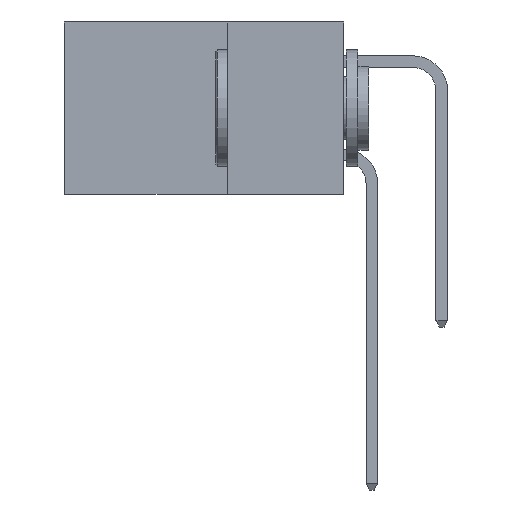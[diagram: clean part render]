
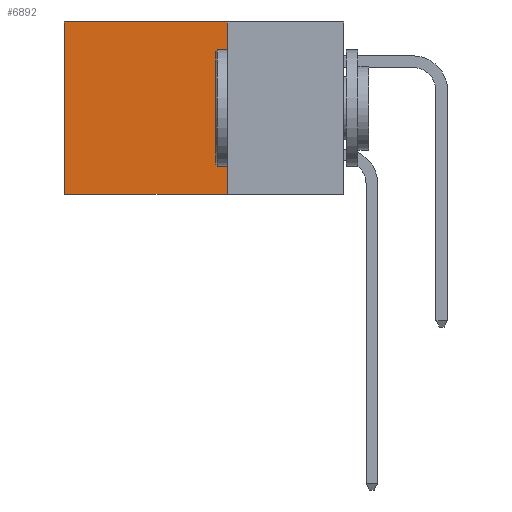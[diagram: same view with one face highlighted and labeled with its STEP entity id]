
A CAD part, left-side view. The second image highlights one B-rep face of the part: STEP entity #6892.
In plain terms, the highlighted planar face has unit normal (-1, 0, 0).
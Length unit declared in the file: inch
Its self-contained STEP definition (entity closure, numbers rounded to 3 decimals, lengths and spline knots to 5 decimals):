
#18 = PLANE ( 'NONE',  #6084 ) ;
#218 = CARTESIAN_POINT ( 'NONE',  ( 0.2615, 0.6, -0.37 ) ) ;
#992 = DIRECTION ( 'NONE',  ( 0., 0., -1. ) ) ;
#1005 = LINE ( 'NONE', #12203, #17346 ) ;
#1094 = EDGE_CURVE ( 'NONE', #1504, #15524, #16859, .T. ) ;
#1504 = VERTEX_POINT ( 'NONE', #9074 ) ;
#2095 = DIRECTION ( 'NONE',  ( 0., 0., -1. ) ) ;
#2265 = ORIENTED_EDGE ( 'NONE', *, *, #1094, .F. ) ;
#3482 = ORIENTED_EDGE ( 'NONE', *, *, #8745, .T. ) ;
#4600 = CARTESIAN_POINT ( 'NONE',  ( 0.2615, 0.25, -0.37 ) ) ;
#5393 = FACE_OUTER_BOUND ( 'NONE', #13277, .T. ) ;
#5619 = CARTESIAN_POINT ( 'NONE',  ( 0.2615, 0.6, -0.37 ) ) ;
#5986 = VECTOR ( 'NONE', #992, 39.37008 ) ;
#6084 = AXIS2_PLACEMENT_3D ( 'NONE', #24496, #14347, #2095 ) ;
#6892 = ADVANCED_FACE ( 'NONE', ( #5393 ), #18, .F. ) ;
#8338 = VERTEX_POINT ( 'NONE', #218 ) ;
#8745 = EDGE_CURVE ( 'NONE', #13707, #8338, #15873, .T. ) ;
#9074 = CARTESIAN_POINT ( 'NONE',  ( 0.2615, 0.25, 0. ) ) ;
#9290 = DIRECTION ( 'NONE',  ( 0., 1., 0. ) ) ;
#12203 = CARTESIAN_POINT ( 'NONE',  ( 0.2615, 0.25, -0.37 ) ) ;
#13277 = EDGE_LOOP ( 'NONE', ( #3482, #20804, #2265, #25917 ) ) ;
#13707 = VERTEX_POINT ( 'NONE', #16728 ) ;
#13932 = EDGE_CURVE ( 'NONE', #1504, #13707, #18506, .T. ) ;
#14347 = DIRECTION ( 'NONE',  ( 1., 0., 0. ) ) ;
#15524 = VERTEX_POINT ( 'NONE', #19948 ) ;
#15873 = LINE ( 'NONE', #5619, #16520 ) ;
#16520 = VECTOR ( 'NONE', #23892, 39.37008 ) ;
#16728 = CARTESIAN_POINT ( 'NONE',  ( 0.2615, 0.6, 0. ) ) ;
#16859 = LINE ( 'NONE', #4600, #5986 ) ;
#17346 = VECTOR ( 'NONE', #26384, 39.37008 ) ;
#18506 = LINE ( 'NONE', #23486, #23899 ) ;
#19948 = CARTESIAN_POINT ( 'NONE',  ( 0.2615, 0.25, -0.37 ) ) ;
#20804 = ORIENTED_EDGE ( 'NONE', *, *, #22814, .F. ) ;
#22814 = EDGE_CURVE ( 'NONE', #15524, #8338, #1005, .T. ) ;
#23486 = CARTESIAN_POINT ( 'NONE',  ( 0.2615, 0.25, 0. ) ) ;
#23892 = DIRECTION ( 'NONE',  ( 0., 0., -1. ) ) ;
#23899 = VECTOR ( 'NONE', #9290, 39.37008 ) ;
#24496 = CARTESIAN_POINT ( 'NONE',  ( 0.2615, 0.25, -0.37 ) ) ;
#25917 = ORIENTED_EDGE ( 'NONE', *, *, #13932, .T. ) ;
#26384 = DIRECTION ( 'NONE',  ( 0., 1., 0. ) ) ;
